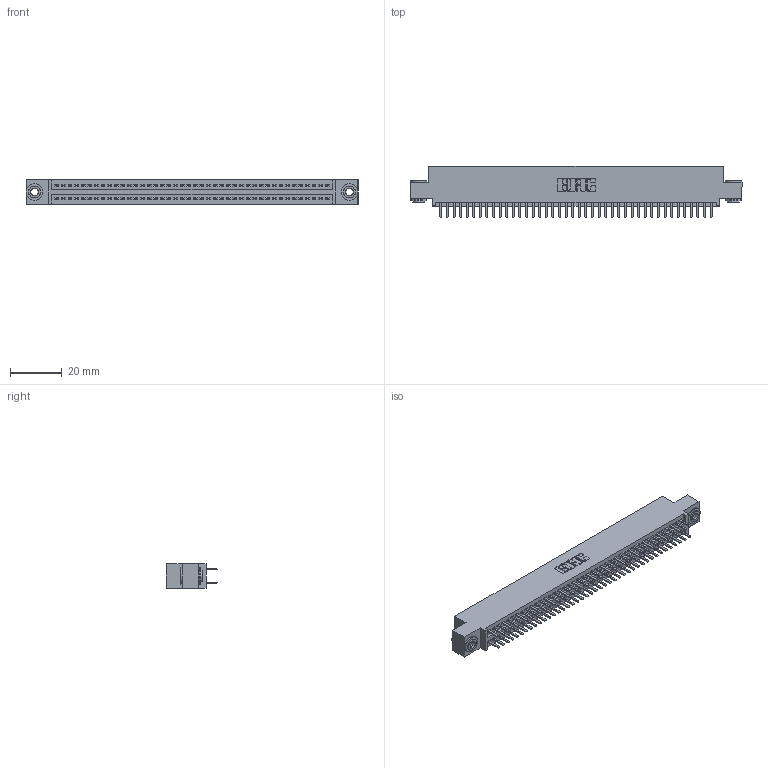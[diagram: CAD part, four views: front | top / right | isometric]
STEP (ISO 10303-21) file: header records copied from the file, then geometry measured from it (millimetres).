
FILE_DESCRIPTION (( 'STEP AP203' ), '1' );
FILE_NAME ('395-084-520-503.STEP', '2019-10-25T08:02:59', ( '' ), ( '' ), 'SwSTEP 2.0', 'SolidWorks 2016', '' );
FILE_SCHEMA (( 'CONFIG_CONTROL_DESIGN' ));
Length unit declared in the file: inch
Products named in the file (4): 345 Part_0.110 Offset - 0.156 Dia-TH; 345-292-001_345-293-120; 345-250-002_345-250-002-102; 395-084-520-503
Assembly tree (87 placements, depth 2):
  395-084-520-503
    345 Part_0.110 Offset - 0.156 Dia-TH
    345-292-001_345-293-120  x84
    345-250-002_345-250-002-102  x2
Bounding box: 127.89 x 19.68 x 9.4 mm (x, y, z)
Volume: 12332.4 mm3; surface area: 18448.5 mm2
Topology: 87 solids, 87 shells, 4704 faces, 13617 edges, 8850 vertices
Faces by surface type: plane 3034, cylinder 1662, cone 8
Entity records: 33850 total; most frequent: CARTESIAN_POINT 5663, ORIENTED_EDGE 5578, DIRECTION 5011, EDGE_CURVE 2789, LINE 2461, VECTOR 2461, VERTEX_POINT 1854, AXIS2_PLACEMENT_3D 1275
